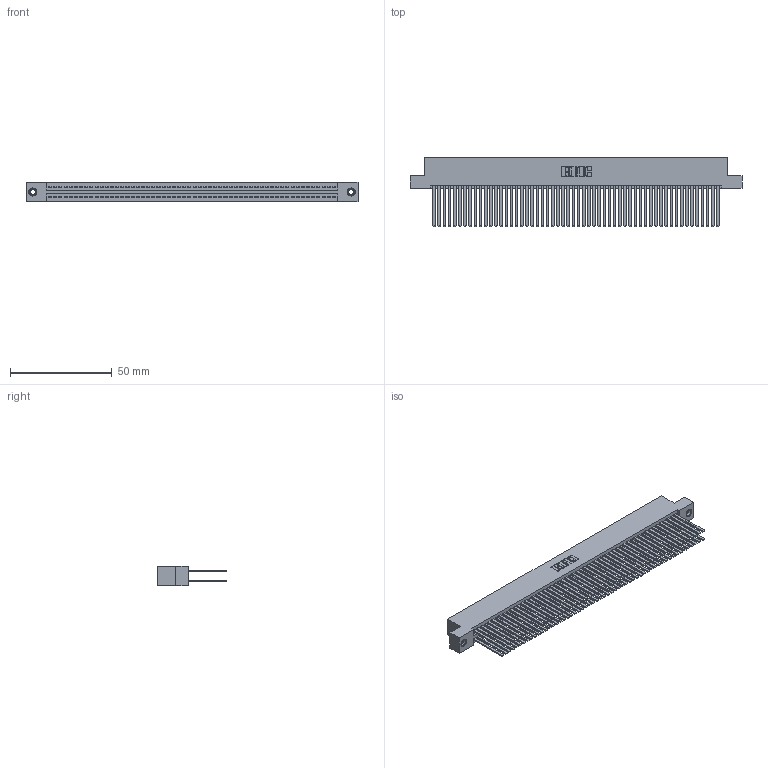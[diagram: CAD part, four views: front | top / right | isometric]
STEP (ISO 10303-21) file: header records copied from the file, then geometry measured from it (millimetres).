
FILE_DESCRIPTION (( 'STEP AP203' ), '1' );
FILE_NAME ('345-112-544-207.STEP', '2019-11-04T22:19:31', ( '' ), ( '' ), 'SwSTEP 2.0', 'SolidWorks 2016', '' );
FILE_SCHEMA (( 'CONFIG_CONTROL_DESIGN' ));
Length unit declared in the file: inch
Products named in the file (4): 345 Part_Flush Mounting Lugs - 0.156 Dia-TI; 345-292-001_345-293-144; 345-250-001_345-250-005-103; 345-112-544-207
Assembly tree (115 placements, depth 2):
  345-112-544-207
    345 Part_Flush Mounting Lugs - 0.156 Dia-TI
    345-292-001_345-293-144  x112
    345-250-001_345-250-005-103  x2
Bounding box: 163.45 x 33.96 x 9.4 mm (x, y, z)
Volume: 17564.1 mm3; surface area: 30863.3 mm2
Topology: 115 solids, 115 shells, 5114 faces, 15149 edges, 9942 vertices
Faces by surface type: plane 3360, cylinder 1738, cone 12, torus 4
Entity records: 43056 total; most frequent: CARTESIAN_POINT 7183, ORIENTED_EDGE 7110, DIRECTION 6341, EDGE_CURVE 3555, LINE 3183, VECTOR 3183, VERTEX_POINT 2364, AXIS2_PLACEMENT_3D 1579
